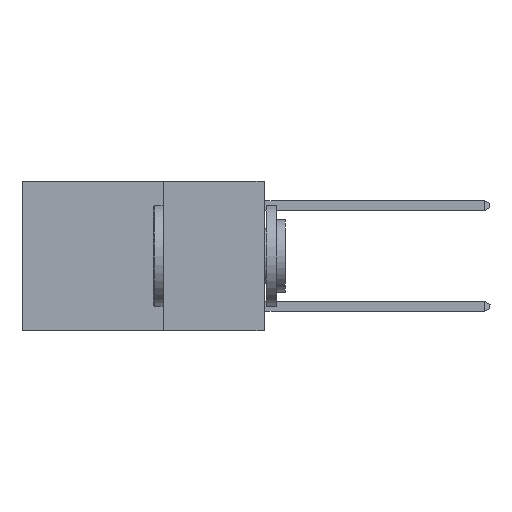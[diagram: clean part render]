
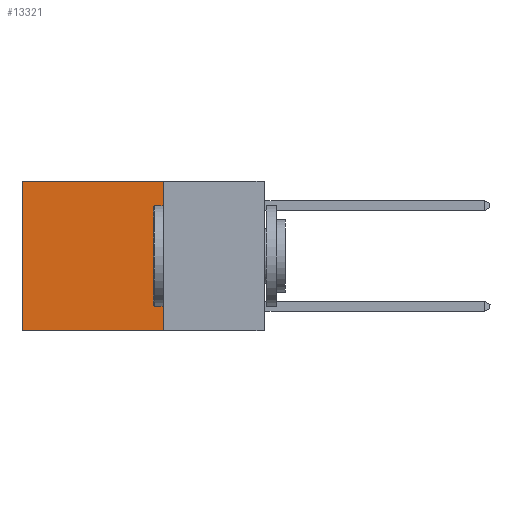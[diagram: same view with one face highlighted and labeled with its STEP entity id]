
A CAD part, left-side view. The second image highlights one B-rep face of the part: STEP entity #13321.
In plain terms, the highlighted planar face has unit normal (-1, 0, 0).
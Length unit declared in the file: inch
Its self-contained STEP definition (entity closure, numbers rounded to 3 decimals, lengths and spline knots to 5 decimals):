
#699 = CARTESIAN_POINT ( 'NONE',  ( 0.2625, 0.25, -0.37 ) ) ;
#973 = CARTESIAN_POINT ( 'NONE',  ( 0.2625, 0.25, 0. ) ) ;
#1280 = CARTESIAN_POINT ( 'NONE',  ( 0.2625, 0.25, 0. ) ) ;
#2016 = ORIENTED_EDGE ( 'NONE', *, *, #18585, .T. ) ;
#2162 = ORIENTED_EDGE ( 'NONE', *, *, #11913, .F. ) ;
#2235 = VECTOR ( 'NONE', #7363, 39.37008 ) ;
#2624 = VERTEX_POINT ( 'NONE', #10754 ) ;
#2819 = DIRECTION ( 'NONE',  ( 0., 0., -1. ) ) ;
#3084 = VERTEX_POINT ( 'NONE', #973 ) ;
#3508 = PLANE ( 'NONE',  #5306 ) ;
#3510 = VECTOR ( 'NONE', #16939, 39.37008 ) ;
#3882 = VECTOR ( 'NONE', #16876, 39.37008 ) ;
#4391 = EDGE_LOOP ( 'NONE', ( #12479, #19806, #2162, #2016 ) ) ;
#4602 = CARTESIAN_POINT ( 'NONE',  ( 0.2625, 0.25, -0.37 ) ) ;
#5076 = DIRECTION ( 'NONE',  ( 1., 0., 0. ) ) ;
#5306 = AXIS2_PLACEMENT_3D ( 'NONE', #12783, #5076, #15828 ) ;
#5932 = EDGE_CURVE ( 'NONE', #10973, #2624, #8030, .T. ) ;
#6485 = FACE_OUTER_BOUND ( 'NONE', #4391, .T. ) ;
#7363 = DIRECTION ( 'NONE',  ( 0., 1., 0. ) ) ;
#7716 = VERTEX_POINT ( 'NONE', #9596 ) ;
#8030 = LINE ( 'NONE', #4602, #3882 ) ;
#8969 = EDGE_CURVE ( 'NONE', #7716, #2624, #15793, .T. ) ;
#9596 = CARTESIAN_POINT ( 'NONE',  ( 0.2625, 0.6, 0. ) ) ;
#10385 = CARTESIAN_POINT ( 'NONE',  ( 0.2625, 0.25, 0. ) ) ;
#10754 = CARTESIAN_POINT ( 'NONE',  ( 0.2625, 0.6, -0.37 ) ) ;
#10973 = VERTEX_POINT ( 'NONE', #699 ) ;
#11132 = LINE ( 'NONE', #1280, #14710 ) ;
#11913 = EDGE_CURVE ( 'NONE', #3084, #10973, #11132, .T. ) ;
#12479 = ORIENTED_EDGE ( 'NONE', *, *, #8969, .T. ) ;
#12783 = CARTESIAN_POINT ( 'NONE',  ( 0.2625, 0.25, 0. ) ) ;
#13321 = ADVANCED_FACE ( 'NONE', ( #6485 ), #3508, .F. ) ;
#14078 = LINE ( 'NONE', #10385, #2235 ) ;
#14710 = VECTOR ( 'NONE', #2819, 39.37008 ) ;
#15417 = CARTESIAN_POINT ( 'NONE',  ( 0.2625, 0.6, 0. ) ) ;
#15793 = LINE ( 'NONE', #15417, #3510 ) ;
#15828 = DIRECTION ( 'NONE',  ( 0., 0., -1. ) ) ;
#16876 = DIRECTION ( 'NONE',  ( 0., 1., 0. ) ) ;
#16939 = DIRECTION ( 'NONE',  ( 0., 0., -1. ) ) ;
#18585 = EDGE_CURVE ( 'NONE', #3084, #7716, #14078, .T. ) ;
#19806 = ORIENTED_EDGE ( 'NONE', *, *, #5932, .F. ) ;
